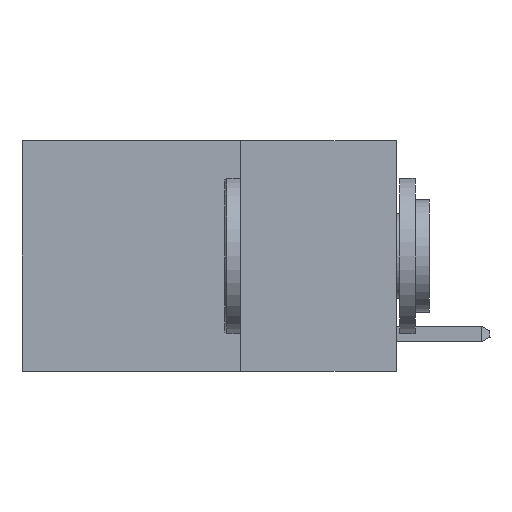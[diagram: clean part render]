
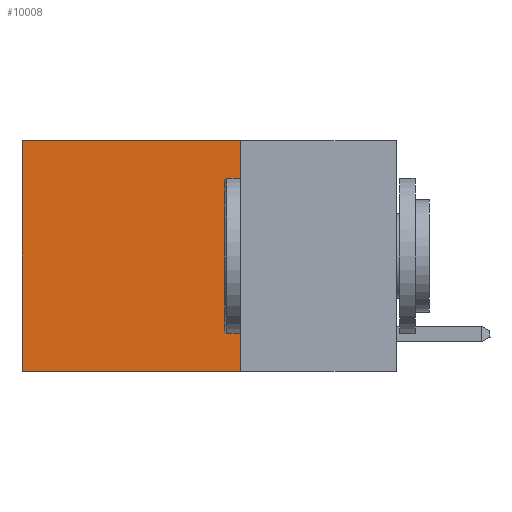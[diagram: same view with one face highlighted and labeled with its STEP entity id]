
A CAD part, left-side view. The second image highlights one B-rep face of the part: STEP entity #10008.
In plain terms, the highlighted planar face has unit normal (-1, 0, 0).
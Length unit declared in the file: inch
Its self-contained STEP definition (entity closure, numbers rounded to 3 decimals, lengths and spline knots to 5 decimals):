
#870 = CARTESIAN_POINT ( 'NONE',  ( 0.2625, 0.6, 0. ) ) ;
#1748 = CARTESIAN_POINT ( 'NONE',  ( 0.2625, 0.6, 0. ) ) ;
#1898 = DIRECTION ( 'NONE',  ( 0., 0., -1. ) ) ;
#1962 = VERTEX_POINT ( 'NONE', #5531 ) ;
#2290 = VECTOR ( 'NONE', #6093, 39.37008 ) ;
#2321 = VECTOR ( 'NONE', #11382, 39.37008 ) ;
#2462 = VERTEX_POINT ( 'NONE', #11598 ) ;
#2567 = CARTESIAN_POINT ( 'NONE',  ( 0.2625, 0.25, -0.37 ) ) ;
#2648 = CARTESIAN_POINT ( 'NONE',  ( 0.2625, 0.6, -0.37 ) ) ;
#2938 = LINE ( 'NONE', #7946, #12117 ) ;
#3757 = ORIENTED_EDGE ( 'NONE', *, *, #4353, .T. ) ;
#3900 = EDGE_CURVE ( 'NONE', #2462, #1962, #2938, .T. ) ;
#4353 = EDGE_CURVE ( 'NONE', #9043, #8035, #14990, .T. ) ;
#4360 = DIRECTION ( 'NONE',  ( 0., 0., -1. ) ) ;
#4625 = EDGE_CURVE ( 'NONE', #1962, #8035, #10246, .T. ) ;
#4897 = AXIS2_PLACEMENT_3D ( 'NONE', #8020, #9177, #1898 ) ;
#5531 = CARTESIAN_POINT ( 'NONE',  ( 0.2625, 0.25, -0.37 ) ) ;
#5751 = EDGE_CURVE ( 'NONE', #2462, #9043, #11506, .T. ) ;
#6093 = DIRECTION ( 'NONE',  ( 0., 1., 0. ) ) ;
#6842 = PLANE ( 'NONE',  #4897 ) ;
#7406 = ORIENTED_EDGE ( 'NONE', *, *, #3900, .F. ) ;
#7518 = DIRECTION ( 'NONE',  ( 0., 1., 0. ) ) ;
#7946 = CARTESIAN_POINT ( 'NONE',  ( 0.2625, 0.25, 0. ) ) ;
#8020 = CARTESIAN_POINT ( 'NONE',  ( 0.2625, 0.25, 0. ) ) ;
#8035 = VERTEX_POINT ( 'NONE', #2648 ) ;
#9043 = VERTEX_POINT ( 'NONE', #870 ) ;
#9177 = DIRECTION ( 'NONE',  ( 1., 0., 0. ) ) ;
#9273 = FACE_OUTER_BOUND ( 'NONE', #12836, .T. ) ;
#9862 = VECTOR ( 'NONE', #7518, 39.37008 ) ;
#10008 = ADVANCED_FACE ( 'NONE', ( #9273 ), #6842, .F. ) ;
#10141 = ORIENTED_EDGE ( 'NONE', *, *, #4625, .F. ) ;
#10246 = LINE ( 'NONE', #2567, #9862 ) ;
#10495 = ORIENTED_EDGE ( 'NONE', *, *, #5751, .T. ) ;
#11382 = DIRECTION ( 'NONE',  ( 0., 0., -1. ) ) ;
#11506 = LINE ( 'NONE', #14252, #2290 ) ;
#11598 = CARTESIAN_POINT ( 'NONE',  ( 0.2625, 0.25, 0. ) ) ;
#12117 = VECTOR ( 'NONE', #4360, 39.37008 ) ;
#12836 = EDGE_LOOP ( 'NONE', ( #3757, #10141, #7406, #10495 ) ) ;
#14252 = CARTESIAN_POINT ( 'NONE',  ( 0.2625, 0.25, 0. ) ) ;
#14990 = LINE ( 'NONE', #1748, #2321 ) ;
